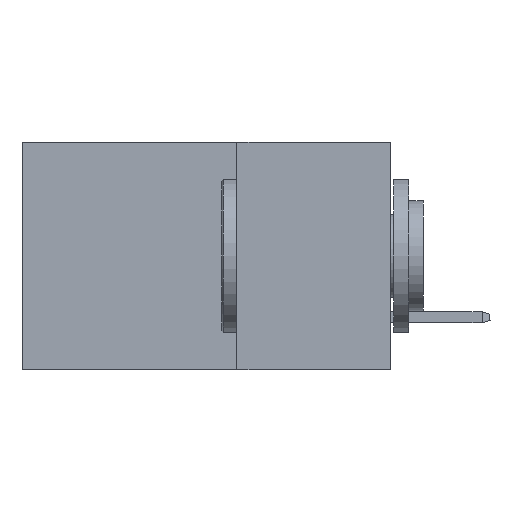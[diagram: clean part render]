
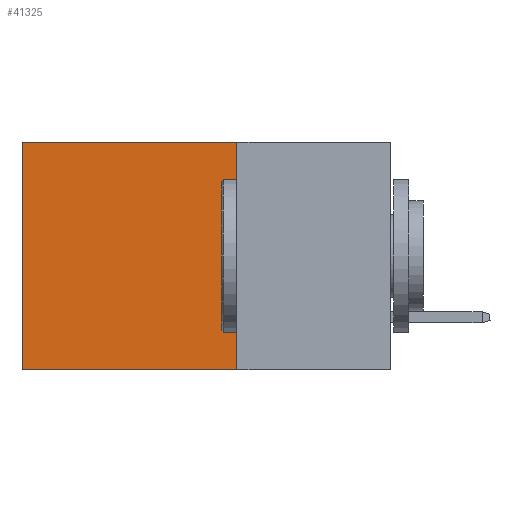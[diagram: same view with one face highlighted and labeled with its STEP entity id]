
A CAD part, left-side view. The second image highlights one B-rep face of the part: STEP entity #41325.
In plain terms, the highlighted planar face has unit normal (-1, 0, 0).
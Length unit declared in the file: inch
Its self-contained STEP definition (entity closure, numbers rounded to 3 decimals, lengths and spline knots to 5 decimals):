
#921 = DIRECTION ( 'NONE',  ( 0., 1., 0. ) ) ;
#1067 = EDGE_CURVE ( 'NONE', #6710, #25797, #19618, .T. ) ;
#2326 = CARTESIAN_POINT ( 'NONE',  ( 0.2875, 0.6, -0.37 ) ) ;
#3788 = LINE ( 'NONE', #43736, #12231 ) ;
#4333 = PLANE ( 'NONE',  #19611 ) ;
#6710 = VERTEX_POINT ( 'NONE', #26245 ) ;
#7953 = DIRECTION ( 'NONE',  ( 1., 0., 0. ) ) ;
#9665 = EDGE_CURVE ( 'NONE', #21559, #22805, #3788, .T. ) ;
#9778 = DIRECTION ( 'NONE',  ( 0., 0., -1. ) ) ;
#10193 = ORIENTED_EDGE ( 'NONE', *, *, #17864, .T. ) ;
#12231 = VECTOR ( 'NONE', #22817, 39.37008 ) ;
#13819 = LINE ( 'NONE', #16271, #25659 ) ;
#15642 = DIRECTION ( 'NONE',  ( 0., 0., -1. ) ) ;
#16271 = CARTESIAN_POINT ( 'NONE',  ( 0.2875, 0.6, 0. ) ) ;
#16422 = ORIENTED_EDGE ( 'NONE', *, *, #9665, .F. ) ;
#17726 = ORIENTED_EDGE ( 'NONE', *, *, #1067, .T. ) ;
#17864 = EDGE_CURVE ( 'NONE', #25797, #22805, #13819, .T. ) ;
#19611 = AXIS2_PLACEMENT_3D ( 'NONE', #22379, #7953, #15642 ) ;
#19618 = LINE ( 'NONE', #43942, #27572 ) ;
#20256 = ORIENTED_EDGE ( 'NONE', *, *, #40298, .F. ) ;
#21559 = VERTEX_POINT ( 'NONE', #23858 ) ;
#22379 = CARTESIAN_POINT ( 'NONE',  ( 0.2875, 0.25, 0. ) ) ;
#22805 = VERTEX_POINT ( 'NONE', #2326 ) ;
#22817 = DIRECTION ( 'NONE',  ( 0., 1., 0. ) ) ;
#23858 = CARTESIAN_POINT ( 'NONE',  ( 0.2875, 0.25, -0.37 ) ) ;
#24687 = CARTESIAN_POINT ( 'NONE',  ( 0.2875, 0.25, 0. ) ) ;
#25659 = VECTOR ( 'NONE', #41884, 39.37008 ) ;
#25792 = EDGE_LOOP ( 'NONE', ( #10193, #16422, #20256, #17726 ) ) ;
#25797 = VERTEX_POINT ( 'NONE', #45993 ) ;
#26245 = CARTESIAN_POINT ( 'NONE',  ( 0.2875, 0.25, 0. ) ) ;
#27572 = VECTOR ( 'NONE', #921, 39.37008 ) ;
#28310 = LINE ( 'NONE', #24687, #42324 ) ;
#40298 = EDGE_CURVE ( 'NONE', #6710, #21559, #28310, .T. ) ;
#41325 = ADVANCED_FACE ( 'NONE', ( #46197 ), #4333, .F. ) ;
#41884 = DIRECTION ( 'NONE',  ( 0., 0., -1. ) ) ;
#42324 = VECTOR ( 'NONE', #9778, 39.37008 ) ;
#43736 = CARTESIAN_POINT ( 'NONE',  ( 0.2875, 0.25, -0.37 ) ) ;
#43942 = CARTESIAN_POINT ( 'NONE',  ( 0.2875, 0.25, 0. ) ) ;
#45993 = CARTESIAN_POINT ( 'NONE',  ( 0.2875, 0.6, 0. ) ) ;
#46197 = FACE_OUTER_BOUND ( 'NONE', #25792, .T. ) ;
